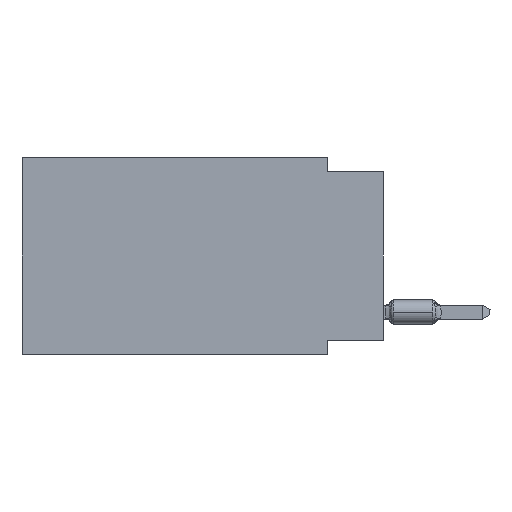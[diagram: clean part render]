
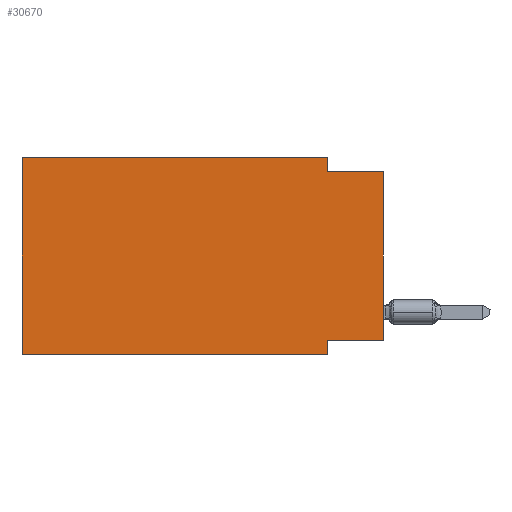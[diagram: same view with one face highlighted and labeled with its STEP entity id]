
A CAD part, left-side view. The second image highlights one B-rep face of the part: STEP entity #30670.
In plain terms, the highlighted planar face has unit normal (-1, 0, 0).
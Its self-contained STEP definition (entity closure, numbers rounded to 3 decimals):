
#2070 = ORIENTED_EDGE ( 'NONE', *, *, #2656, .F. ) ;
#2656 = EDGE_CURVE ( 'NONE', #16610, #5135, #23133, .T. ) ;
#3565 = ORIENTED_EDGE ( 'NONE', *, *, #36257, .F. ) ;
#3649 = VERTEX_POINT ( 'NONE', #28596 ) ;
#4169 = VERTEX_POINT ( 'NONE', #38743 ) ;
#4361 = ORIENTED_EDGE ( 'NONE', *, *, #35471, .F. ) ;
#5135 = VERTEX_POINT ( 'NONE', #5579 ) ;
#5356 = CARTESIAN_POINT ( 'NONE',  ( 0., 16.383, -8.89 ) ) ;
#5571 = LINE ( 'NONE', #27100, #23941 ) ;
#5579 = CARTESIAN_POINT ( 'NONE',  ( 0., 0., -0.635 ) ) ;
#6182 = DIRECTION ( 'NONE',  ( 0., 0., 1. ) ) ;
#7631 = DIRECTION ( 'NONE',  ( 1., 0., 0. ) ) ;
#7669 = DIRECTION ( 'NONE',  ( 0., -1., 0. ) ) ;
#7880 = LINE ( 'NONE', #30459, #16806 ) ;
#8484 = DIRECTION ( 'NONE',  ( 0., -1., 0. ) ) ;
#8646 = CARTESIAN_POINT ( 'NONE',  ( 0., 2.54, 0. ) ) ;
#9327 = ORIENTED_EDGE ( 'NONE', *, *, #37727, .F. ) ;
#9795 = CARTESIAN_POINT ( 'NONE',  ( 0., 16.383, 0. ) ) ;
#10593 = ORIENTED_EDGE ( 'NONE', *, *, #21211, .T. ) ;
#10925 = DIRECTION ( 'NONE',  ( 0., 0., 1. ) ) ;
#11142 = LINE ( 'NONE', #8646, #11409 ) ;
#11400 = LINE ( 'NONE', #5356, #32450 ) ;
#11409 = VECTOR ( 'NONE', #24313, 1000. ) ;
#11517 = ORIENTED_EDGE ( 'NONE', *, *, #14037, .F. ) ;
#11622 = VERTEX_POINT ( 'NONE', #28211 ) ;
#12425 = VECTOR ( 'NONE', #7669, 1000. ) ;
#14037 = EDGE_CURVE ( 'NONE', #11622, #35187, #7880, .T. ) ;
#14751 = VECTOR ( 'NONE', #10925, 1000. ) ;
#16610 = VERTEX_POINT ( 'NONE', #18748 ) ;
#16668 = EDGE_LOOP ( 'NONE', ( #10593, #2070, #4361, #24941, #9327, #30976, #11517, #3565 ) ) ;
#16806 = VECTOR ( 'NONE', #26926, 1000. ) ;
#18748 = CARTESIAN_POINT ( 'NONE',  ( 0., 2.54, -0.635 ) ) ;
#20996 = VERTEX_POINT ( 'NONE', #29636 ) ;
#21016 = DIRECTION ( 'NONE',  ( 0., 1., 0. ) ) ;
#21203 = DIRECTION ( 'NONE',  ( 0., -1., 0. ) ) ;
#21211 = EDGE_CURVE ( 'NONE', #3649, #5135, #34825, .T. ) ;
#23133 = LINE ( 'NONE', #26699, #12425 ) ;
#23941 = VECTOR ( 'NONE', #8484, 1000. ) ;
#24313 = DIRECTION ( 'NONE',  ( 0., 0., -1. ) ) ;
#24941 = ORIENTED_EDGE ( 'NONE', *, *, #33090, .F. ) ;
#26029 = PLANE ( 'NONE',  #29144 ) ;
#26699 = CARTESIAN_POINT ( 'NONE',  ( 0., 0., -0.635 ) ) ;
#26827 = LINE ( 'NONE', #39541, #14751 ) ;
#26926 = DIRECTION ( 'NONE',  ( 0., 0., -1. ) ) ;
#27100 = CARTESIAN_POINT ( 'NONE',  ( 0., 16.383, 0. ) ) ;
#28211 = CARTESIAN_POINT ( 'NONE',  ( 0., 2.54, -8.255 ) ) ;
#28282 = EDGE_CURVE ( 'NONE', #20996, #35187, #11400, .T. ) ;
#28596 = CARTESIAN_POINT ( 'NONE',  ( 0., 0., -8.255 ) ) ;
#28824 = VERTEX_POINT ( 'NONE', #9795 ) ;
#29144 = AXIS2_PLACEMENT_3D ( 'NONE', #35650, #7631, #39582 ) ;
#29636 = CARTESIAN_POINT ( 'NONE',  ( 0., 16.383, -8.89 ) ) ;
#30094 = VECTOR ( 'NONE', #6182, 1000. ) ;
#30459 = CARTESIAN_POINT ( 'NONE',  ( 0., 2.54, -8.89 ) ) ;
#30670 = ADVANCED_FACE ( 'NONE', ( #36266 ), #26029, .F. ) ;
#30870 = CARTESIAN_POINT ( 'NONE',  ( 0., 0., 0. ) ) ;
#30976 = ORIENTED_EDGE ( 'NONE', *, *, #28282, .T. ) ;
#32450 = VECTOR ( 'NONE', #21203, 1000. ) ;
#33090 = EDGE_CURVE ( 'NONE', #28824, #4169, #5571, .T. ) ;
#34218 = LINE ( 'NONE', #40238, #40725 ) ;
#34825 = LINE ( 'NONE', #30870, #30094 ) ;
#35187 = VERTEX_POINT ( 'NONE', #35436 ) ;
#35436 = CARTESIAN_POINT ( 'NONE',  ( 0., 2.54, -8.89 ) ) ;
#35471 = EDGE_CURVE ( 'NONE', #4169, #16610, #11142, .T. ) ;
#35650 = CARTESIAN_POINT ( 'NONE',  ( 0., 16.383, 0. ) ) ;
#36257 = EDGE_CURVE ( 'NONE', #3649, #11622, #34218, .T. ) ;
#36266 = FACE_OUTER_BOUND ( 'NONE', #16668, .T. ) ;
#37727 = EDGE_CURVE ( 'NONE', #20996, #28824, #26827, .T. ) ;
#38743 = CARTESIAN_POINT ( 'NONE',  ( 0., 2.54, 0. ) ) ;
#39541 = CARTESIAN_POINT ( 'NONE',  ( 0., 16.383, 0. ) ) ;
#39582 = DIRECTION ( 'NONE',  ( 0., 0., -1. ) ) ;
#40238 = CARTESIAN_POINT ( 'NONE',  ( 0., 0., -8.255 ) ) ;
#40725 = VECTOR ( 'NONE', #21016, 1000. ) ;
